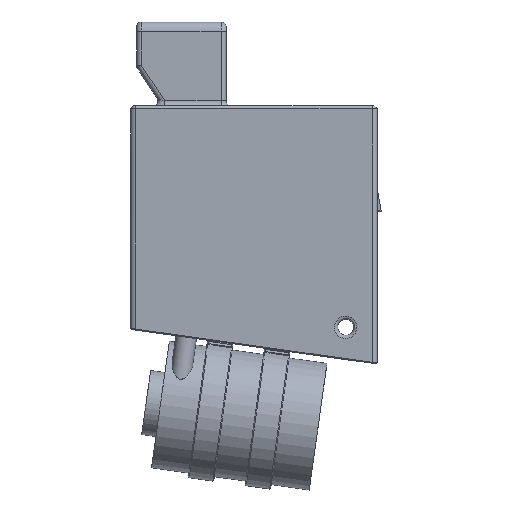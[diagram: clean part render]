
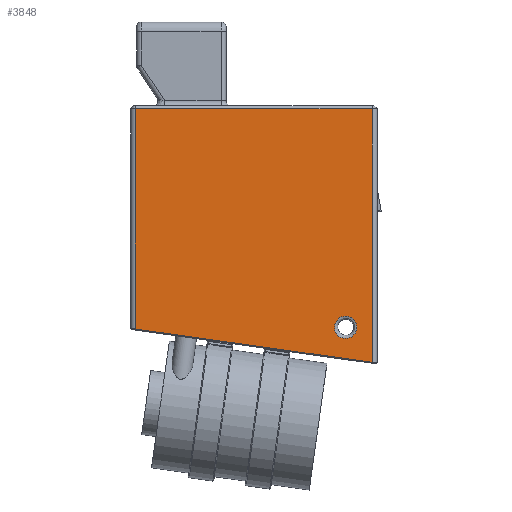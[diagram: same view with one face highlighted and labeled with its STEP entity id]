
A CAD part, left-side view. The second image highlights one B-rep face of the part: STEP entity #3848.
In plain terms, the highlighted planar face has unit normal (-1, 0.025, 0).
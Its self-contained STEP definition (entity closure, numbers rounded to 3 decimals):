
#51=ELLIPSE('',#4174,3.501,3.5);
#191=B_SPLINE_CURVE_WITH_KNOTS('',3,(#6228,#6229,#6230,#6231),
 .UNSPECIFIED.,.F.,.F.,(4,4),(-1.546,-1.518),
 .UNSPECIFIED.);
#231=FACE_BOUND('',#631,.T.);
#264=PLANE('',#4177);
#355=FACE_OUTER_BOUND('',#630,.T.);
#630=EDGE_LOOP('',(#2674,#2675,#2676,#2677,#2678));
#631=EDGE_LOOP('',(#2679));
#904=LINE('',#6224,#1146);
#905=LINE('',#6226,#1147);
#906=LINE('',#6233,#1148);
#907=LINE('',#6234,#1149);
#1146=VECTOR('',#4793,10.);
#1147=VECTOR('',#4794,10.);
#1148=VECTOR('',#4795,10.);
#1149=VECTOR('',#4796,10.);
#1665=VERTEX_POINT('',#6212);
#1668=VERTEX_POINT('',#6222);
#1669=VERTEX_POINT('',#6223);
#1670=VERTEX_POINT('',#6225);
#1671=VERTEX_POINT('',#6227);
#1672=VERTEX_POINT('',#6232);
#2029=EDGE_CURVE('',#1665,#1665,#51,.T.);
#2032=EDGE_CURVE('',#1668,#1669,#904,.T.);
#2033=EDGE_CURVE('',#1670,#1668,#905,.T.);
#2034=EDGE_CURVE('',#1671,#1670,#191,.T.);
#2035=EDGE_CURVE('',#1672,#1671,#906,.T.);
#2036=EDGE_CURVE('',#1669,#1672,#907,.T.);
#2674=ORIENTED_EDGE('',*,*,#2032,.F.);
#2675=ORIENTED_EDGE('',*,*,#2033,.F.);
#2676=ORIENTED_EDGE('',*,*,#2034,.F.);
#2677=ORIENTED_EDGE('',*,*,#2035,.F.);
#2678=ORIENTED_EDGE('',*,*,#2036,.F.);
#2679=ORIENTED_EDGE('',*,*,#2029,.F.);
#3848=ADVANCED_FACE('',(#355,#231),#264,.T.);
#4174=AXIS2_PLACEMENT_3D('',#6216,#4784,#4785);
#4177=AXIS2_PLACEMENT_3D('',#6221,#4791,#4792);
#4784=DIRECTION('center_axis',(-1.,0.025,0.));
#4785=DIRECTION('ref_axis',(0.025,1.,0.));
#4791=DIRECTION('center_axis',(-1.,0.025,0.));
#4792=DIRECTION('ref_axis',(-0.025,-1.,0.));
#4793=DIRECTION('',(-0.025,-1.,0.));
#4794=DIRECTION('',(0.,0.,1.));
#4795=DIRECTION('',(0.025,0.99,0.139));
#4796=DIRECTION('',(0.,0.,-1.));
#6212=CARTESIAN_POINT('',(0.364,6.525,11.504));
#6216=CARTESIAN_POINT('Origin',(0.452,10.025,11.504));
#6221=CARTESIAN_POINT('Origin',(2.15,77.445,0.));
#6222=CARTESIAN_POINT('',(2.108,75.788,79.8));
#6223=CARTESIAN_POINT('',(0.244,1.738,79.8));
#6224=CARTESIAN_POINT('',(1.666,58.226,79.8));
#6225=CARTESIAN_POINT('',(2.108,75.788,10.954));
#6226=CARTESIAN_POINT('',(2.108,75.788,0.));
#6227=CARTESIAN_POINT('',(2.107,75.746,10.948));
#6228=CARTESIAN_POINT('Ctrl Pts',(2.107,75.746,10.948));
#6229=CARTESIAN_POINT('Ctrl Pts',(2.108,75.76,10.95));
#6230=CARTESIAN_POINT('Ctrl Pts',(2.108,75.774,10.952));
#6231=CARTESIAN_POINT('Ctrl Pts',(2.108,75.788,10.954));
#6232=CARTESIAN_POINT('',(0.244,1.738,0.547));
#6233=CARTESIAN_POINT('',(2.133,76.782,11.094));
#6234=CARTESIAN_POINT('',(0.244,1.738,0.));
